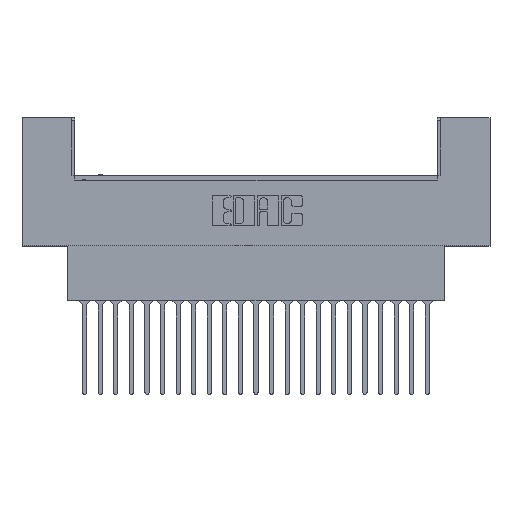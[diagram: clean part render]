
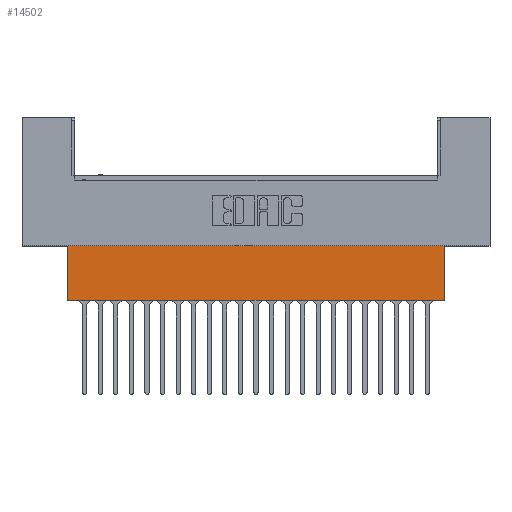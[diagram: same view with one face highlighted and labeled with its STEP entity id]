
A CAD part, top view. The second image highlights one B-rep face of the part: STEP entity #14502.
In plain terms, the highlighted planar face has unit normal (0, 0, 1).
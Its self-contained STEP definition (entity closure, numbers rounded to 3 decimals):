
#373 = VERTEX_POINT ( 'NONE', #29395 ) ;
#1749 = VECTOR ( 'NONE', #24225, 1000. ) ;
#2068 = DIRECTION ( 'NONE',  ( -1., 0., 0. ) ) ;
#2595 = DIRECTION ( 'NONE',  ( 0., 0., -1. ) ) ;
#3622 = AXIS2_PLACEMENT_3D ( 'NONE', #25909, #2595, #16670 ) ;
#4729 = LINE ( 'NONE', #23399, #9406 ) ;
#6823 = ORIENTED_EDGE ( 'NONE', *, *, #29211, .F. ) ;
#8152 = CARTESIAN_POINT ( 'NONE',  ( 7.468, 0., -3.962 ) ) ;
#8559 = CARTESIAN_POINT ( 'NONE',  ( 76.352, -8.814, -3.962 ) ) ;
#8777 = VECTOR ( 'NONE', #29072, 1000. ) ;
#9406 = VECTOR ( 'NONE', #14660, 1000. ) ;
#10206 = EDGE_LOOP ( 'NONE', ( #6823, #17623, #23345, #24589 ) ) ;
#10939 = LINE ( 'NONE', #13067, #8777 ) ;
#11971 = PLANE ( 'NONE',  #3622 ) ;
#12574 = LINE ( 'NONE', #8559, #1749 ) ;
#13067 = CARTESIAN_POINT ( 'NONE',  ( 7.468, -8.814, -3.962 ) ) ;
#13829 = VERTEX_POINT ( 'NONE', #28296 ) ;
#14071 = LINE ( 'NONE', #20573, #19472 ) ;
#14502 = ADVANCED_FACE ( 'NONE', ( #29099 ), #11971, .F. ) ;
#14660 = DIRECTION ( 'NONE',  ( 0., -1., 0. ) ) ;
#16670 = DIRECTION ( 'NONE',  ( 0., 1., 0. ) ) ;
#17346 = VERTEX_POINT ( 'NONE', #26779 ) ;
#17623 = ORIENTED_EDGE ( 'NONE', *, *, #27934, .F. ) ;
#18003 = EDGE_CURVE ( 'NONE', #373, #21851, #10939, .T. ) ;
#19472 = VECTOR ( 'NONE', #2068, 1000. ) ;
#20573 = CARTESIAN_POINT ( 'NONE',  ( 76.352, 0., -3.962 ) ) ;
#21851 = VERTEX_POINT ( 'NONE', #8152 ) ;
#22307 = EDGE_CURVE ( 'NONE', #13829, #21851, #14071, .T. ) ;
#23345 = ORIENTED_EDGE ( 'NONE', *, *, #22307, .T. ) ;
#23399 = CARTESIAN_POINT ( 'NONE',  ( 68.885, -8.814, -3.962 ) ) ;
#24225 = DIRECTION ( 'NONE',  ( -1., 0., 0. ) ) ;
#24589 = ORIENTED_EDGE ( 'NONE', *, *, #18003, .F. ) ;
#25909 = CARTESIAN_POINT ( 'NONE',  ( 76.352, 0., -3.962 ) ) ;
#26779 = CARTESIAN_POINT ( 'NONE',  ( 68.885, -8.814, -3.962 ) ) ;
#27934 = EDGE_CURVE ( 'NONE', #13829, #17346, #4729, .T. ) ;
#28296 = CARTESIAN_POINT ( 'NONE',  ( 68.885, 0., -3.962 ) ) ;
#29072 = DIRECTION ( 'NONE',  ( 0., 1., 0. ) ) ;
#29099 = FACE_OUTER_BOUND ( 'NONE', #10206, .T. ) ;
#29211 = EDGE_CURVE ( 'NONE', #17346, #373, #12574, .T. ) ;
#29395 = CARTESIAN_POINT ( 'NONE',  ( 7.468, -8.814, -3.962 ) ) ;
